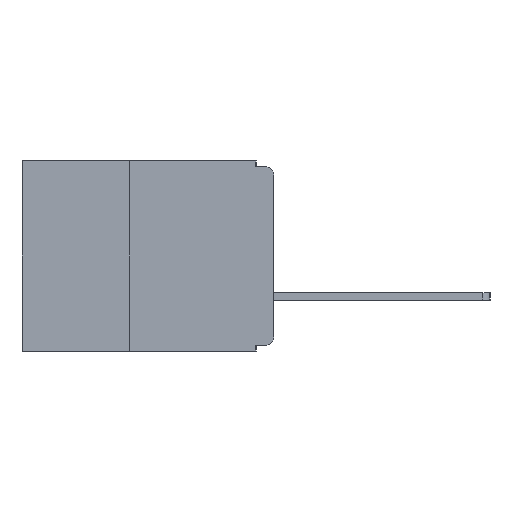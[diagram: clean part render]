
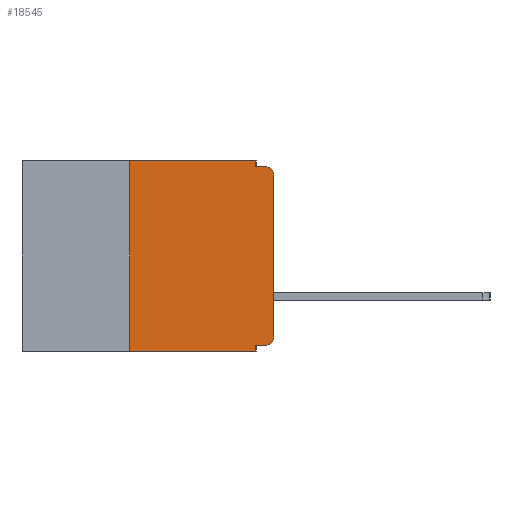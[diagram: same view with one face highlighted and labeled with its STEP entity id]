
A CAD part, left-side view. The second image highlights one B-rep face of the part: STEP entity #18545.
In plain terms, the highlighted planar face has unit normal (-1, 0, 0).
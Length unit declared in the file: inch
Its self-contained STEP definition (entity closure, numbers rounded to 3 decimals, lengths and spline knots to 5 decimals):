
#87 = VERTEX_POINT ( 'NONE', #8340 ) ;
#187 = CARTESIAN_POINT ( 'NONE',  ( 0., 0., -0.305 ) ) ;
#252 = CARTESIAN_POINT ( 'NONE',  ( 0., 0.015, -0.01 ) ) ;
#538 = VERTEX_POINT ( 'NONE', #20221 ) ;
#1007 = EDGE_CURVE ( 'NONE', #16003, #18548, #4793, .T. ) ;
#1779 = VECTOR ( 'NONE', #7207, 39.37008 ) ;
#1910 = CARTESIAN_POINT ( 'NONE',  ( 0., 0.031, -0.01 ) ) ;
#2135 = VERTEX_POINT ( 'NONE', #187 ) ;
#2329 = DIRECTION ( 'NONE',  ( -1., 0., 0. ) ) ;
#2341 = PLANE ( 'NONE',  #16949 ) ;
#2725 = VECTOR ( 'NONE', #9494, 39.37008 ) ;
#2784 = LINE ( 'NONE', #16728, #1779 ) ;
#3069 = EDGE_CURVE ( 'NONE', #5721, #2135, #11021, .T. ) ;
#3257 = DIRECTION ( 'NONE',  ( 0., -1., 0. ) ) ;
#3488 = DIRECTION ( 'NONE',  ( 0., -1., 0. ) ) ;
#3508 = LINE ( 'NONE', #11408, #7362 ) ;
#3563 = AXIS2_PLACEMENT_3D ( 'NONE', #18446, #6267, #6221 ) ;
#3844 = ORIENTED_EDGE ( 'NONE', *, *, #17159, .T. ) ;
#3991 = DIRECTION ( 'NONE',  ( 0., 0., -1. ) ) ;
#4522 = EDGE_CURVE ( 'NONE', #5721, #87, #3508, .T. ) ;
#4793 = LINE ( 'NONE', #9104, #12831 ) ;
#4900 = EDGE_CURVE ( 'NONE', #2135, #538, #17491, .T. ) ;
#4912 = CARTESIAN_POINT ( 'NONE',  ( 0., 0.25, -0.33 ) ) ;
#5144 = LINE ( 'NONE', #14463, #12177 ) ;
#5413 = EDGE_CURVE ( 'NONE', #18548, #19000, #7100, .T. ) ;
#5576 = LINE ( 'NONE', #10198, #13556 ) ;
#5655 = CARTESIAN_POINT ( 'NONE',  ( 0., 0.031, 0. ) ) ;
#5656 = ORIENTED_EDGE ( 'NONE', *, *, #1007, .F. ) ;
#5721 = VERTEX_POINT ( 'NONE', #10324 ) ;
#5727 = CARTESIAN_POINT ( 'NONE',  ( 0., 0.25, -0.33 ) ) ;
#6221 = DIRECTION ( 'NONE',  ( 0., 0., -1. ) ) ;
#6267 = DIRECTION ( 'NONE',  ( -1., 0., 0. ) ) ;
#6557 = DIRECTION ( 'NONE',  ( 0., 0., 1. ) ) ;
#6678 = ORIENTED_EDGE ( 'NONE', *, *, #17686, .F. ) ;
#6926 = ORIENTED_EDGE ( 'NONE', *, *, #8931, .T. ) ;
#7100 = LINE ( 'NONE', #18845, #2725 ) ;
#7207 = DIRECTION ( 'NONE',  ( 0., 0., -1. ) ) ;
#7339 = VECTOR ( 'NONE', #6557, 39.37008 ) ;
#7362 = VECTOR ( 'NONE', #11268, 39.37008 ) ;
#8340 = CARTESIAN_POINT ( 'NONE',  ( 0., 0.031, -0.32 ) ) ;
#8931 = EDGE_CURVE ( 'NONE', #538, #14461, #19013, .T. ) ;
#9104 = CARTESIAN_POINT ( 'NONE',  ( 0., 0.437, 0. ) ) ;
#9330 = EDGE_CURVE ( 'NONE', #19000, #14461, #5144, .T. ) ;
#9375 = VERTEX_POINT ( 'NONE', #16104 ) ;
#9485 = ORIENTED_EDGE ( 'NONE', *, *, #5413, .F. ) ;
#9494 = DIRECTION ( 'NONE',  ( 0., 0., -1. ) ) ;
#10198 = CARTESIAN_POINT ( 'NONE',  ( 0., 0.437, -0.33 ) ) ;
#10324 = CARTESIAN_POINT ( 'NONE',  ( 0., 0.015, -0.32 ) ) ;
#10479 = CARTESIAN_POINT ( 'NONE',  ( 0., 0.437, 0. ) ) ;
#10745 = ORIENTED_EDGE ( 'NONE', *, *, #3069, .T. ) ;
#10876 = AXIS2_PLACEMENT_3D ( 'NONE', #12043, #2329, #13583 ) ;
#11021 = CIRCLE ( 'NONE', #3563, 0.015 ) ;
#11268 = DIRECTION ( 'NONE',  ( 0., 1., 0. ) ) ;
#11408 = CARTESIAN_POINT ( 'NONE',  ( 0., 0., -0.32 ) ) ;
#11560 = FACE_OUTER_BOUND ( 'NONE', #14280, .T. ) ;
#11765 = DIRECTION ( 'NONE',  ( 0., -1., 0. ) ) ;
#12043 = CARTESIAN_POINT ( 'NONE',  ( 0., 0.015, -0.025 ) ) ;
#12177 = VECTOR ( 'NONE', #3257, 39.37008 ) ;
#12691 = CARTESIAN_POINT ( 'NONE',  ( 0., 0.25, 0. ) ) ;
#12831 = VECTOR ( 'NONE', #3488, 39.37008 ) ;
#12918 = ORIENTED_EDGE ( 'NONE', *, *, #4900, .T. ) ;
#13408 = ORIENTED_EDGE ( 'NONE', *, *, #4522, .F. ) ;
#13556 = VECTOR ( 'NONE', #11765, 39.37008 ) ;
#13583 = DIRECTION ( 'NONE',  ( 0., 0., -1. ) ) ;
#13592 = DIRECTION ( 'NONE',  ( 1., 0., 0. ) ) ;
#13829 = VECTOR ( 'NONE', #17256, 39.37008 ) ;
#14280 = EDGE_LOOP ( 'NONE', ( #12918, #6926, #19490, #9485, #5656, #6678, #3844, #16582, #13408, #10745 ) ) ;
#14461 = VERTEX_POINT ( 'NONE', #252 ) ;
#14463 = CARTESIAN_POINT ( 'NONE',  ( 0., 0., -0.01 ) ) ;
#15214 = EDGE_CURVE ( 'NONE', #87, #9375, #2784, .T. ) ;
#16003 = VERTEX_POINT ( 'NONE', #12691 ) ;
#16104 = CARTESIAN_POINT ( 'NONE',  ( 0., 0.031, -0.33 ) ) ;
#16582 = ORIENTED_EDGE ( 'NONE', *, *, #15214, .F. ) ;
#16728 = CARTESIAN_POINT ( 'NONE',  ( 0., 0.031, -0.33 ) ) ;
#16949 = AXIS2_PLACEMENT_3D ( 'NONE', #10479, #13592, #3991 ) ;
#17159 = EDGE_CURVE ( 'NONE', #20633, #9375, #5576, .T. ) ;
#17256 = DIRECTION ( 'NONE',  ( 0., 0., 1. ) ) ;
#17330 = CARTESIAN_POINT ( 'NONE',  ( 0., 0., 0. ) ) ;
#17491 = LINE ( 'NONE', #17330, #13829 ) ;
#17686 = EDGE_CURVE ( 'NONE', #20633, #16003, #19867, .T. ) ;
#18446 = CARTESIAN_POINT ( 'NONE',  ( 0., 0.015, -0.305 ) ) ;
#18545 = ADVANCED_FACE ( 'NONE', ( #11560 ), #2341, .F. ) ;
#18548 = VERTEX_POINT ( 'NONE', #5655 ) ;
#18845 = CARTESIAN_POINT ( 'NONE',  ( 0., 0.031, 0. ) ) ;
#19000 = VERTEX_POINT ( 'NONE', #1910 ) ;
#19013 = CIRCLE ( 'NONE', #10876, 0.015 ) ;
#19490 = ORIENTED_EDGE ( 'NONE', *, *, #9330, .F. ) ;
#19867 = LINE ( 'NONE', #4912, #7339 ) ;
#20221 = CARTESIAN_POINT ( 'NONE',  ( 0., 0., -0.025 ) ) ;
#20633 = VERTEX_POINT ( 'NONE', #5727 ) ;
